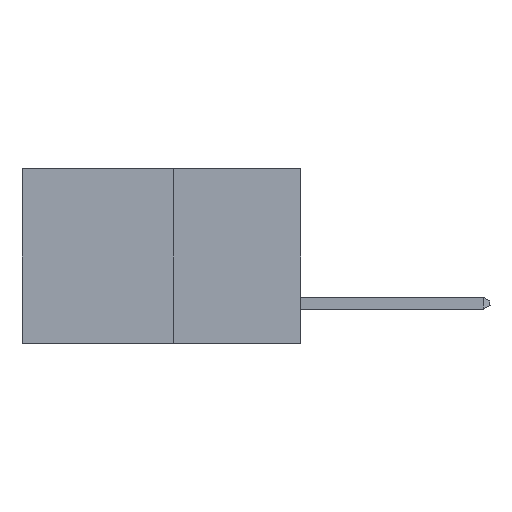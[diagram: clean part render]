
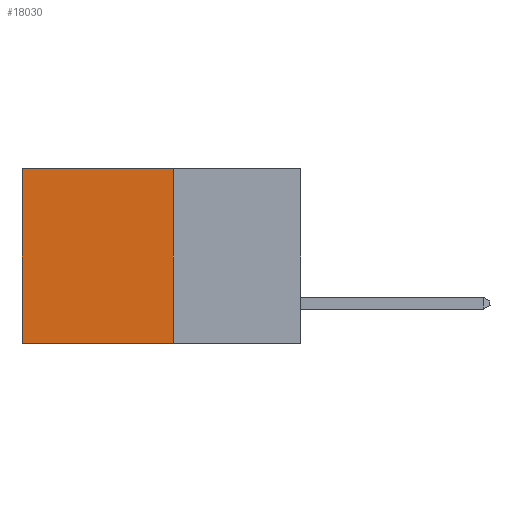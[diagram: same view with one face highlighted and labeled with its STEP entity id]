
A CAD part, left-side view. The second image highlights one B-rep face of the part: STEP entity #18030.
In plain terms, the highlighted planar face has unit normal (-1, 0, 0).
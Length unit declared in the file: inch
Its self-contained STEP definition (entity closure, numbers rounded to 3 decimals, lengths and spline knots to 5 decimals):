
#1134 = CARTESIAN_POINT ( 'NONE',  ( 0.277, 0.27, 0. ) ) ;
#1424 = CARTESIAN_POINT ( 'NONE',  ( 0.277, 0.27, -0.37 ) ) ;
#1581 = DIRECTION ( 'NONE',  ( 0., 1., 0. ) ) ;
#3114 = DIRECTION ( 'NONE',  ( 0., 0., -1. ) ) ;
#4681 = FACE_OUTER_BOUND ( 'NONE', #15863, .T. ) ;
#5105 = VECTOR ( 'NONE', #8026, 39.37008 ) ;
#5212 = VECTOR ( 'NONE', #5874, 39.37008 ) ;
#5556 = DIRECTION ( 'NONE',  ( 0., 1., 0. ) ) ;
#5649 = LINE ( 'NONE', #1134, #13264 ) ;
#5874 = DIRECTION ( 'NONE',  ( 0., 0., -1. ) ) ;
#6629 = ORIENTED_EDGE ( 'NONE', *, *, #6775, .F. ) ;
#6775 = EDGE_CURVE ( 'NONE', #18930, #9543, #8948, .T. ) ;
#7171 = VERTEX_POINT ( 'NONE', #17216 ) ;
#7849 = ORIENTED_EDGE ( 'NONE', *, *, #10887, .T. ) ;
#8026 = DIRECTION ( 'NONE',  ( 0., 0., -1. ) ) ;
#8689 = CARTESIAN_POINT ( 'NONE',  ( 0.277, 0.59, -0.37 ) ) ;
#8948 = LINE ( 'NONE', #1424, #17946 ) ;
#9397 = LINE ( 'NONE', #8689, #5105 ) ;
#9543 = VERTEX_POINT ( 'NONE', #17213 ) ;
#9550 = PLANE ( 'NONE',  #10292 ) ;
#10292 = AXIS2_PLACEMENT_3D ( 'NONE', #11203, #12834, #3114 ) ;
#10887 = EDGE_CURVE ( 'NONE', #12559, #7171, #5649, .T. ) ;
#11203 = CARTESIAN_POINT ( 'NONE',  ( 0.277, 0.27, -0.37 ) ) ;
#11678 = EDGE_CURVE ( 'NONE', #7171, #9543, #9397, .T. ) ;
#12333 = CARTESIAN_POINT ( 'NONE',  ( 0.277, 0.27, -0.37 ) ) ;
#12559 = VERTEX_POINT ( 'NONE', #16151 ) ;
#12834 = DIRECTION ( 'NONE',  ( 1., 0., 0. ) ) ;
#13264 = VECTOR ( 'NONE', #5556, 39.37008 ) ;
#13811 = LINE ( 'NONE', #12333, #5212 ) ;
#14656 = ORIENTED_EDGE ( 'NONE', *, *, #11678, .T. ) ;
#15863 = EDGE_LOOP ( 'NONE', ( #14656, #6629, #20521, #7849 ) ) ;
#16151 = CARTESIAN_POINT ( 'NONE',  ( 0.277, 0.27, 0. ) ) ;
#17074 = EDGE_CURVE ( 'NONE', #12559, #18930, #13811, .T. ) ;
#17213 = CARTESIAN_POINT ( 'NONE',  ( 0.277, 0.59, -0.37 ) ) ;
#17216 = CARTESIAN_POINT ( 'NONE',  ( 0.277, 0.59, 0. ) ) ;
#17946 = VECTOR ( 'NONE', #1581, 39.37008 ) ;
#18030 = ADVANCED_FACE ( 'NONE', ( #4681 ), #9550, .F. ) ;
#18361 = CARTESIAN_POINT ( 'NONE',  ( 0.277, 0.27, -0.37 ) ) ;
#18930 = VERTEX_POINT ( 'NONE', #18361 ) ;
#20521 = ORIENTED_EDGE ( 'NONE', *, *, #17074, .F. ) ;
